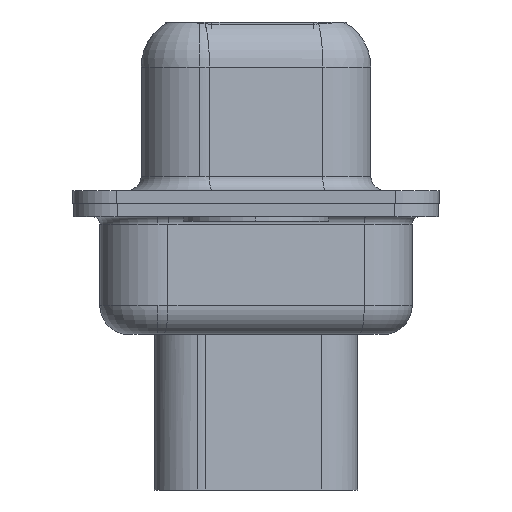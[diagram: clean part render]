
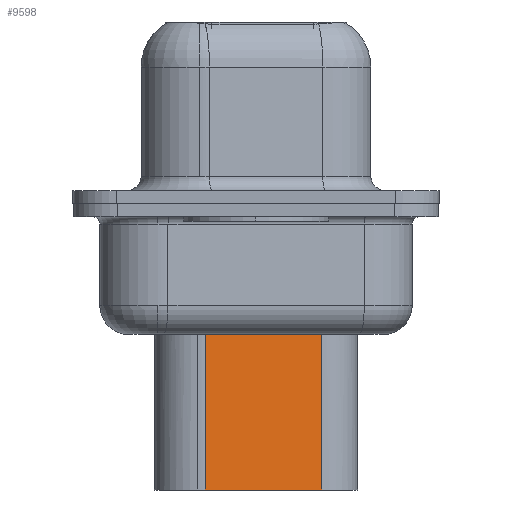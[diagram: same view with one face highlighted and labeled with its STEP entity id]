
A CAD part, left-side view. The second image highlights one B-rep face of the part: STEP entity #9598.
In plain terms, the highlighted planar face has unit normal (-0.985, -0.174, 0).
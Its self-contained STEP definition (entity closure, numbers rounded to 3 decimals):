
#30 = DIRECTION ( 'NONE',  ( -0.985, -0.174, 0. ) ) ;
#253 = FACE_OUTER_BOUND ( 'NONE', #22129, .T. ) ;
#1771 = CARTESIAN_POINT ( 'NONE',  ( 4.519, 1.74, -9.85 ) ) ;
#2729 = CARTESIAN_POINT ( 'NONE',  ( 4.348, 2.709, -3.975 ) ) ;
#2822 = VECTOR ( 'NONE', #9978, 1000. ) ;
#3459 = ORIENTED_EDGE ( 'NONE', *, *, #8200, .T. ) ;
#4275 = CARTESIAN_POINT ( 'NONE',  ( 5.224, -2.26, -9.85 ) ) ;
#4840 = EDGE_CURVE ( 'NONE', #22107, #8366, #8722, .T. ) ;
#5122 = CARTESIAN_POINT ( 'NONE',  ( 4.519, 1.74, -3.1 ) ) ;
#5131 = ORIENTED_EDGE ( 'NONE', *, *, #4840, .F. ) ;
#7412 = VERTEX_POINT ( 'NONE', #18576 ) ;
#8200 = EDGE_CURVE ( 'NONE', #7412, #23234, #12705, .T. ) ;
#8366 = VERTEX_POINT ( 'NONE', #4275 ) ;
#8722 = LINE ( 'NONE', #19902, #8743 ) ;
#8743 = VECTOR ( 'NONE', #9211, 1000. ) ;
#8768 = VECTOR ( 'NONE', #19594, 1000. ) ;
#9211 = DIRECTION ( 'NONE',  ( 0., 0., -1. ) ) ;
#9598 = ADVANCED_FACE ( 'NONE', ( #253 ), #13084, .T. ) ;
#9978 = DIRECTION ( 'NONE',  ( -0.174, 0.985, 0. ) ) ;
#11244 = EDGE_CURVE ( 'NONE', #22107, #7412, #15086, .T. ) ;
#12234 = LINE ( 'NONE', #1771, #23049 ) ;
#12705 = LINE ( 'NONE', #5122, #8768 ) ;
#13084 = PLANE ( 'NONE',  #23148 ) ;
#15086 = LINE ( 'NONE', #2729, #2822 ) ;
#16621 = ORIENTED_EDGE ( 'NONE', *, *, #22103, .F. ) ;
#17676 = DIRECTION ( 'NONE',  ( -0.174, 0.985, 0. ) ) ;
#18180 = DIRECTION ( 'NONE',  ( 0.174, -0.985, 0. ) ) ;
#18576 = CARTESIAN_POINT ( 'NONE',  ( 4.519, 1.74, -3.975 ) ) ;
#19594 = DIRECTION ( 'NONE',  ( 0., 0., -1. ) ) ;
#19902 = CARTESIAN_POINT ( 'NONE',  ( 5.224, -2.26, -3.1 ) ) ;
#19956 = CARTESIAN_POINT ( 'NONE',  ( 4.519, 1.74, -9.85 ) ) ;
#20329 = CARTESIAN_POINT ( 'NONE',  ( 4.519, 1.74, -3.1 ) ) ;
#22103 = EDGE_CURVE ( 'NONE', #8366, #23234, #12234, .T. ) ;
#22107 = VERTEX_POINT ( 'NONE', #23409 ) ;
#22129 = EDGE_LOOP ( 'NONE', ( #5131, #22391, #3459, #16621 ) ) ;
#22391 = ORIENTED_EDGE ( 'NONE', *, *, #11244, .T. ) ;
#23049 = VECTOR ( 'NONE', #17676, 1000. ) ;
#23148 = AXIS2_PLACEMENT_3D ( 'NONE', #20329, #30, #18180 ) ;
#23234 = VERTEX_POINT ( 'NONE', #19956 ) ;
#23409 = CARTESIAN_POINT ( 'NONE',  ( 5.224, -2.26, -3.975 ) ) ;
